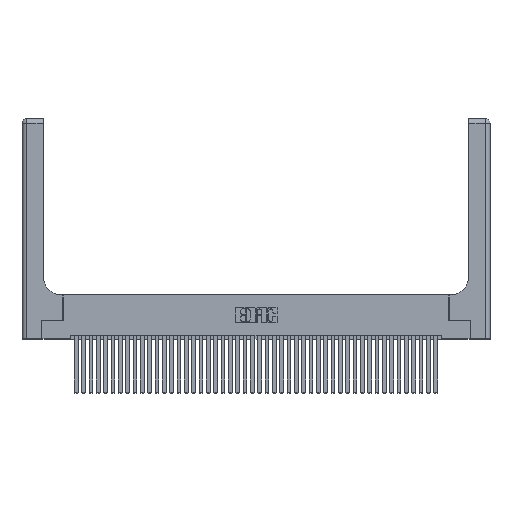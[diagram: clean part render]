
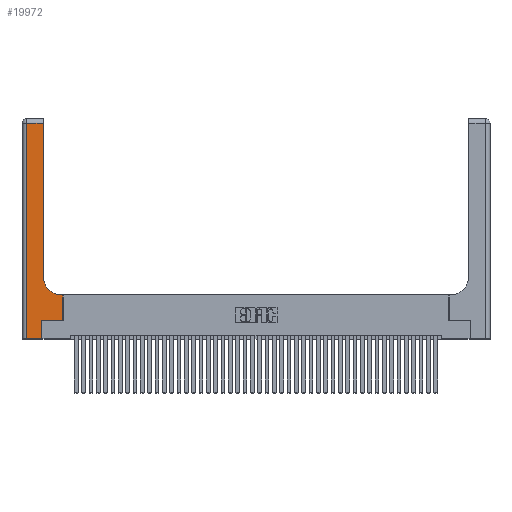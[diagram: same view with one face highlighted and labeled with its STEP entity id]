
A CAD part, top view. The second image highlights one B-rep face of the part: STEP entity #19972.
In plain terms, the highlighted planar face has unit normal (0, 0, 1).
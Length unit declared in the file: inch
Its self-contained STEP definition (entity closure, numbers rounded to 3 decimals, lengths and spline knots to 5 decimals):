
#628 = EDGE_CURVE ( 'NONE', #10505, #14697, #7533, .T. ) ;
#3637 = VERTEX_POINT ( 'NONE', #23472 ) ;
#3735 = CARTESIAN_POINT ( 'NONE',  ( 0., 0., 0.37 ) ) ;
#3880 = EDGE_CURVE ( 'NONE', #6614, #3637, #38951, .T. ) ;
#4928 = DIRECTION ( 'NONE',  ( 0., 0., -1. ) ) ;
#5177 = ORIENTED_EDGE ( 'NONE', *, *, #10467, .T. ) ;
#5393 = VECTOR ( 'NONE', #40354, 39.37008 ) ;
#5442 = VERTEX_POINT ( 'NONE', #30837 ) ;
#5962 = DIRECTION ( 'NONE',  ( 0., 1., 0. ) ) ;
#6095 = ORIENTED_EDGE ( 'NONE', *, *, #11195, .T. ) ;
#6573 = EDGE_CURVE ( 'NONE', #30200, #20155, #9564, .T. ) ;
#6614 = VERTEX_POINT ( 'NONE', #9675 ) ;
#6876 = LINE ( 'NONE', #36485, #42155 ) ;
#7143 = VECTOR ( 'NONE', #35682, 39.37008 ) ;
#7533 = LINE ( 'NONE', #12663, #24217 ) ;
#8228 = PLANE ( 'NONE',  #34032 ) ;
#9389 = CARTESIAN_POINT ( 'NONE',  ( 0.269, 0., 0.37 ) ) ;
#9564 = LINE ( 'NONE', #9389, #33962 ) ;
#9675 = CARTESIAN_POINT ( 'NONE',  ( 0.5585, 0.6, 0.37 ) ) ;
#9789 = DIRECTION ( 'NONE',  ( 0., 1., 0. ) ) ;
#10467 = EDGE_CURVE ( 'NONE', #11291, #6614, #23760, .T. ) ;
#10505 = VERTEX_POINT ( 'NONE', #43037 ) ;
#10985 = CARTESIAN_POINT ( 'NONE',  ( 0.5585, 0.25, 0.37 ) ) ;
#11195 = EDGE_CURVE ( 'NONE', #20101, #30200, #24211, .T. ) ;
#11291 = VERTEX_POINT ( 'NONE', #10985 ) ;
#11386 = EDGE_CURVE ( 'NONE', #3637, #10505, #25752, .T. ) ;
#11426 = CARTESIAN_POINT ( 'NONE',  ( 0.5415, 0.85, 0.37 ) ) ;
#11847 = DIRECTION ( 'NONE',  ( -1., 0., 0. ) ) ;
#12240 = ORIENTED_EDGE ( 'NONE', *, *, #29395, .T. ) ;
#12242 = CARTESIAN_POINT ( 'NONE',  ( 0.06, 3., 0.37 ) ) ;
#12663 = CARTESIAN_POINT ( 'NONE',  ( 0.2915, 3., 0.37 ) ) ;
#12814 = LINE ( 'NONE', #12242, #38198 ) ;
#13556 = CARTESIAN_POINT ( 'NONE',  ( 0.2915, 2.94, 0.37 ) ) ;
#14697 = VERTEX_POINT ( 'NONE', #13556 ) ;
#14799 = DIRECTION ( 'NONE',  ( 1., 0., 0. ) ) ;
#14968 = VECTOR ( 'NONE', #9789, 39.37008 ) ;
#15870 = CARTESIAN_POINT ( 'NONE',  ( 0., 2.94, 0.37 ) ) ;
#16017 = DIRECTION ( 'NONE',  ( 0., 1., 0. ) ) ;
#16033 = EDGE_CURVE ( 'NONE', #20155, #11291, #6876, .T. ) ;
#18150 = ORIENTED_EDGE ( 'NONE', *, *, #3880, .T. ) ;
#18596 = ORIENTED_EDGE ( 'NONE', *, *, #16033, .T. ) ;
#19972 = ADVANCED_FACE ( 'NONE', ( #29204 ), #8228, .F. ) ;
#20101 = VERTEX_POINT ( 'NONE', #28897 ) ;
#20155 = VERTEX_POINT ( 'NONE', #39223 ) ;
#21638 = CARTESIAN_POINT ( 'NONE',  ( 0., 3., 0.37 ) ) ;
#23167 = DIRECTION ( 'NONE',  ( 1., 0., 0. ) ) ;
#23438 = VECTOR ( 'NONE', #11847, 39.37008 ) ;
#23472 = CARTESIAN_POINT ( 'NONE',  ( 0.5415, 0.6, 0.37 ) ) ;
#23760 = LINE ( 'NONE', #42758, #14968 ) ;
#23850 = LINE ( 'NONE', #15870, #7143 ) ;
#24211 = LINE ( 'NONE', #3735, #5393 ) ;
#24217 = VECTOR ( 'NONE', #16017, 39.37008 ) ;
#25752 = CIRCLE ( 'NONE', #27028, 0.25 ) ;
#27028 = AXIS2_PLACEMENT_3D ( 'NONE', #11426, #34616, #14799 ) ;
#28320 = DIRECTION ( 'NONE',  ( -1., 0., 0. ) ) ;
#28897 = CARTESIAN_POINT ( 'NONE',  ( 0.06, 0., 0.37 ) ) ;
#29028 = ORIENTED_EDGE ( 'NONE', *, *, #11386, .T. ) ;
#29204 = FACE_OUTER_BOUND ( 'NONE', #32902, .T. ) ;
#29395 = EDGE_CURVE ( 'NONE', #14697, #5442, #23850, .T. ) ;
#29543 = ORIENTED_EDGE ( 'NONE', *, *, #33044, .T. ) ;
#30200 = VERTEX_POINT ( 'NONE', #39623 ) ;
#30837 = CARTESIAN_POINT ( 'NONE',  ( 0.06, 2.94, 0.37 ) ) ;
#32111 = DIRECTION ( 'NONE',  ( 0., -1., 0. ) ) ;
#32902 = EDGE_LOOP ( 'NONE', ( #41591, #12240, #29543, #6095, #38527, #18596, #5177, #18150, #29028 ) ) ;
#33044 = EDGE_CURVE ( 'NONE', #5442, #20101, #12814, .T. ) ;
#33962 = VECTOR ( 'NONE', #5962, 39.37008 ) ;
#34032 = AXIS2_PLACEMENT_3D ( 'NONE', #21638, #4928, #28320 ) ;
#34616 = DIRECTION ( 'NONE',  ( 0., 0., -1. ) ) ;
#35038 = CARTESIAN_POINT ( 'NONE',  ( 0.2915, 0.6, 0.37 ) ) ;
#35682 = DIRECTION ( 'NONE',  ( -1., 0., 0. ) ) ;
#36485 = CARTESIAN_POINT ( 'NONE',  ( 0.269, 0.25, 0.37 ) ) ;
#38198 = VECTOR ( 'NONE', #32111, 39.37008 ) ;
#38527 = ORIENTED_EDGE ( 'NONE', *, *, #6573, .T. ) ;
#38951 = LINE ( 'NONE', #35038, #23438 ) ;
#39223 = CARTESIAN_POINT ( 'NONE',  ( 0.269, 0.25, 0.37 ) ) ;
#39623 = CARTESIAN_POINT ( 'NONE',  ( 0.269, 0., 0.37 ) ) ;
#40354 = DIRECTION ( 'NONE',  ( 1., 0., 0. ) ) ;
#41591 = ORIENTED_EDGE ( 'NONE', *, *, #628, .T. ) ;
#42155 = VECTOR ( 'NONE', #23167, 39.37008 ) ;
#42758 = CARTESIAN_POINT ( 'NONE',  ( 0.5585, 0.25, 0.37 ) ) ;
#43037 = CARTESIAN_POINT ( 'NONE',  ( 0.2915, 0.85, 0.37 ) ) ;
